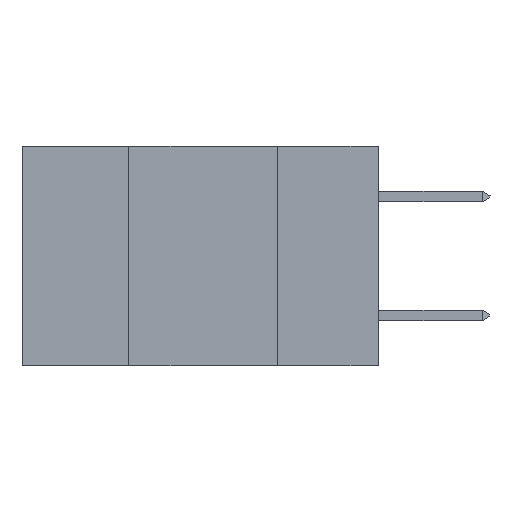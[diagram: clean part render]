
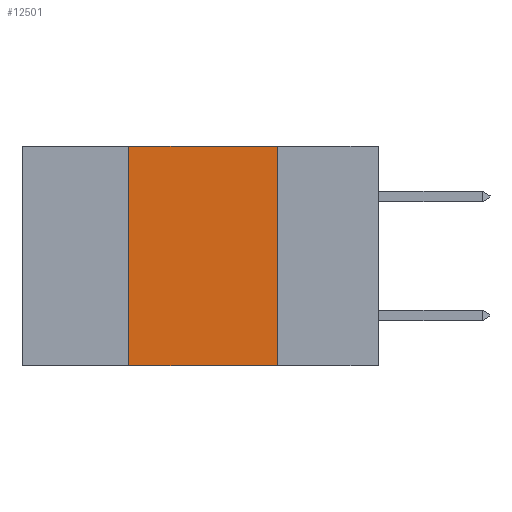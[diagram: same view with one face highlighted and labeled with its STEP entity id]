
A CAD part, left-side view. The second image highlights one B-rep face of the part: STEP entity #12501.
In plain terms, the highlighted planar face has unit normal (-1, 0, 0).
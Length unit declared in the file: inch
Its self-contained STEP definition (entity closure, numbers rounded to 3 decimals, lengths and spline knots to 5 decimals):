
#532 = VERTEX_POINT ( 'NONE', #1956 ) ;
#544 = CARTESIAN_POINT ( 'NONE',  ( 0., 0.6, 0. ) ) ;
#1005 = CARTESIAN_POINT ( 'NONE',  ( 0., 0.6, 0. ) ) ;
#1266 = ORIENTED_EDGE ( 'NONE', *, *, #1342, .F. ) ;
#1342 = EDGE_CURVE ( 'NONE', #532, #11292, #11729, .T. ) ;
#1384 = LINE ( 'NONE', #6924, #10295 ) ;
#1956 = CARTESIAN_POINT ( 'NONE',  ( 0., 0.42, 0. ) ) ;
#2110 = EDGE_CURVE ( 'NONE', #6215, #532, #10497, .T. ) ;
#2228 = PLANE ( 'NONE',  #13815 ) ;
#2367 = LINE ( 'NONE', #4559, #11542 ) ;
#4559 = CARTESIAN_POINT ( 'NONE',  ( 0., 0.6, -0.37 ) ) ;
#4855 = CARTESIAN_POINT ( 'NONE',  ( 0., 0.17, 0. ) ) ;
#5458 = ORIENTED_EDGE ( 'NONE', *, *, #2110, .F. ) ;
#5553 = EDGE_CURVE ( 'NONE', #6215, #13637, #2367, .T. ) ;
#5768 = DIRECTION ( 'NONE',  ( 0., -1., 0. ) ) ;
#6215 = VERTEX_POINT ( 'NONE', #8348 ) ;
#6834 = FACE_OUTER_BOUND ( 'NONE', #7078, .T. ) ;
#6924 = CARTESIAN_POINT ( 'NONE',  ( 0., 0.17, -0.37 ) ) ;
#7078 = EDGE_LOOP ( 'NONE', ( #14207, #1266, #5458, #13991 ) ) ;
#7423 = CARTESIAN_POINT ( 'NONE',  ( 0., 0.42, -0.37 ) ) ;
#7735 = VECTOR ( 'NONE', #13950, 39.37008 ) ;
#8236 = VECTOR ( 'NONE', #11588, 39.37008 ) ;
#8348 = CARTESIAN_POINT ( 'NONE',  ( 0., 0.42, -0.37 ) ) ;
#8805 = CARTESIAN_POINT ( 'NONE',  ( 0., 0.17, -0.37 ) ) ;
#8826 = DIRECTION ( 'NONE',  ( 1., 0., 0. ) ) ;
#10295 = VECTOR ( 'NONE', #11380, 39.37008 ) ;
#10404 = EDGE_CURVE ( 'NONE', #11292, #13637, #1384, .T. ) ;
#10497 = LINE ( 'NONE', #7423, #8236 ) ;
#11292 = VERTEX_POINT ( 'NONE', #4855 ) ;
#11380 = DIRECTION ( 'NONE',  ( 0., 0., -1. ) ) ;
#11542 = VECTOR ( 'NONE', #5768, 39.37008 ) ;
#11588 = DIRECTION ( 'NONE',  ( 0., 0., 1. ) ) ;
#11729 = LINE ( 'NONE', #544, #7735 ) ;
#12501 = ADVANCED_FACE ( 'NONE', ( #6834 ), #2228, .F. ) ;
#13448 = DIRECTION ( 'NONE',  ( 0., 0., -1. ) ) ;
#13637 = VERTEX_POINT ( 'NONE', #8805 ) ;
#13815 = AXIS2_PLACEMENT_3D ( 'NONE', #1005, #8826, #13448 ) ;
#13950 = DIRECTION ( 'NONE',  ( 0., -1., 0. ) ) ;
#13991 = ORIENTED_EDGE ( 'NONE', *, *, #5553, .T. ) ;
#14207 = ORIENTED_EDGE ( 'NONE', *, *, #10404, .F. ) ;
